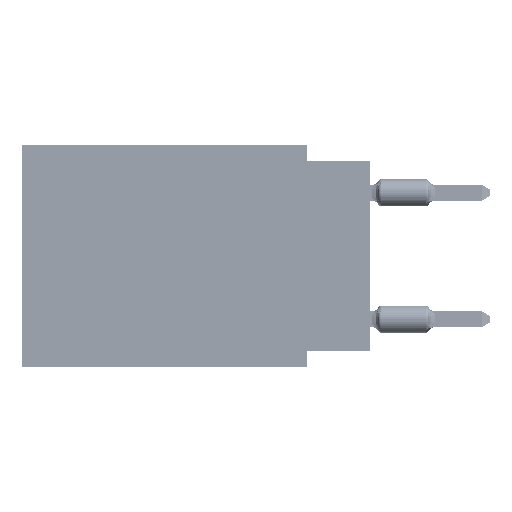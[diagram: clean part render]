
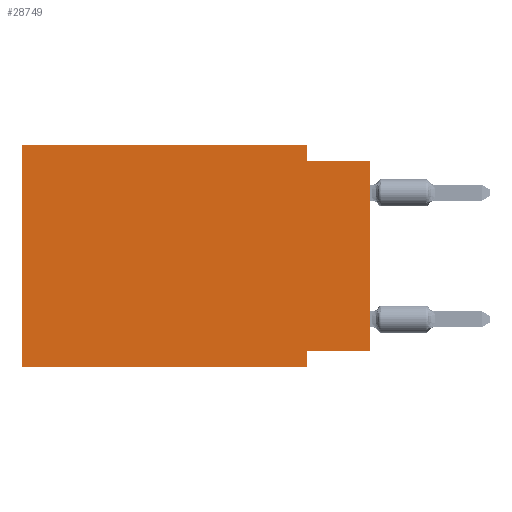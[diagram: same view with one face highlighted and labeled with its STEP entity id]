
A CAD part, left-side view. The second image highlights one B-rep face of the part: STEP entity #28749.
In plain terms, the highlighted planar face has unit normal (-1, 0, 0).
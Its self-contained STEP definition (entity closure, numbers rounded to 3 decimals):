
#2673 = CARTESIAN_POINT ( 'NONE',  ( 0., 13.97, 0. ) ) ;
#3300 = CARTESIAN_POINT ( 'NONE',  ( 0., 2.54, -8.89 ) ) ;
#5452 = LINE ( 'NONE', #49306, #40307 ) ;
#6065 = CARTESIAN_POINT ( 'NONE',  ( 0., 0., -8.255 ) ) ;
#8276 = EDGE_CURVE ( 'NONE', #54910, #14964, #117105, .T. ) ;
#8331 = VECTOR ( 'NONE', #71181, 1000. ) ;
#9939 = EDGE_CURVE ( 'NONE', #44845, #18019, #48872, .T. ) ;
#13936 = DIRECTION ( 'NONE',  ( 0., 0., -1. ) ) ;
#14964 = VERTEX_POINT ( 'NONE', #2673 ) ;
#15237 = CARTESIAN_POINT ( 'NONE',  ( 0., 2.54, -8.89 ) ) ;
#16315 = VERTEX_POINT ( 'NONE', #67379 ) ;
#18019 = VERTEX_POINT ( 'NONE', #29750 ) ;
#19288 = CARTESIAN_POINT ( 'NONE',  ( 0., 0., -0.635 ) ) ;
#24327 = PLANE ( 'NONE',  #94145 ) ;
#25534 = CARTESIAN_POINT ( 'NONE',  ( 0., 0., 0. ) ) ;
#26233 = VERTEX_POINT ( 'NONE', #15237 ) ;
#27404 = DIRECTION ( 'NONE',  ( 0., 1., 0. ) ) ;
#28749 = ADVANCED_FACE ( 'NONE', ( #51570 ), #24327, .F. ) ;
#29750 = CARTESIAN_POINT ( 'NONE',  ( 0., 0., -0.635 ) ) ;
#32771 = CARTESIAN_POINT ( 'NONE',  ( 0., 13.97, -8.89 ) ) ;
#34827 = ORIENTED_EDGE ( 'NONE', *, *, #89122, .F. ) ;
#35045 = CARTESIAN_POINT ( 'NONE',  ( 0., 13.97, 0. ) ) ;
#36717 = DIRECTION ( 'NONE',  ( 0., 0., 1. ) ) ;
#38510 = ORIENTED_EDGE ( 'NONE', *, *, #9939, .F. ) ;
#38607 = LINE ( 'NONE', #47521, #50872 ) ;
#40307 = VECTOR ( 'NONE', #59360, 1000. ) ;
#40900 = CARTESIAN_POINT ( 'NONE',  ( 0., 13.97, 0. ) ) ;
#44845 = VERTEX_POINT ( 'NONE', #47089 ) ;
#47089 = CARTESIAN_POINT ( 'NONE',  ( 0., 2.54, -0.635 ) ) ;
#47521 = CARTESIAN_POINT ( 'NONE',  ( 0., 0., -8.255 ) ) ;
#47622 = EDGE_CURVE ( 'NONE', #99064, #44845, #5452, .T. ) ;
#48186 = ORIENTED_EDGE ( 'NONE', *, *, #61670, .T. ) ;
#48872 = LINE ( 'NONE', #19288, #99717 ) ;
#49306 = CARTESIAN_POINT ( 'NONE',  ( 0., 2.54, 0. ) ) ;
#50872 = VECTOR ( 'NONE', #27404, 1000. ) ;
#51570 = FACE_OUTER_BOUND ( 'NONE', #85907, .T. ) ;
#52399 = VECTOR ( 'NONE', #115671, 1000. ) ;
#53425 = LINE ( 'NONE', #35045, #8331 ) ;
#54518 = LINE ( 'NONE', #25534, #69589 ) ;
#54910 = VERTEX_POINT ( 'NONE', #92592 ) ;
#59360 = DIRECTION ( 'NONE',  ( 0., 0., -1. ) ) ;
#61670 = EDGE_CURVE ( 'NONE', #88846, #18019, #54518, .T. ) ;
#63228 = CARTESIAN_POINT ( 'NONE',  ( 0., 13.97, 0. ) ) ;
#66443 = ORIENTED_EDGE ( 'NONE', *, *, #90180, .F. ) ;
#67121 = VECTOR ( 'NONE', #98190, 1000. ) ;
#67379 = CARTESIAN_POINT ( 'NONE',  ( 0., 2.54, -8.255 ) ) ;
#69329 = DIRECTION ( 'NONE',  ( 0., 0., -1. ) ) ;
#69589 = VECTOR ( 'NONE', #36717, 1000. ) ;
#70048 = ORIENTED_EDGE ( 'NONE', *, *, #96653, .F. ) ;
#71181 = DIRECTION ( 'NONE',  ( 0., -1., 0. ) ) ;
#74978 = LINE ( 'NONE', #3300, #89832 ) ;
#85907 = EDGE_LOOP ( 'NONE', ( #48186, #38510, #97736, #34827, #115506, #116827, #66443, #70048 ) ) ;
#88054 = CARTESIAN_POINT ( 'NONE',  ( 0., 2.54, 0. ) ) ;
#88846 = VERTEX_POINT ( 'NONE', #6065 ) ;
#89122 = EDGE_CURVE ( 'NONE', #14964, #99064, #53425, .T. ) ;
#89832 = VECTOR ( 'NONE', #13936, 1000. ) ;
#90180 = EDGE_CURVE ( 'NONE', #16315, #26233, #74978, .T. ) ;
#92592 = CARTESIAN_POINT ( 'NONE',  ( 0., 13.97, -8.89 ) ) ;
#94145 = AXIS2_PLACEMENT_3D ( 'NONE', #40900, #104291, #69329 ) ;
#96653 = EDGE_CURVE ( 'NONE', #88846, #16315, #38607, .T. ) ;
#97736 = ORIENTED_EDGE ( 'NONE', *, *, #47622, .F. ) ;
#98190 = DIRECTION ( 'NONE',  ( 0., 0., 1. ) ) ;
#99064 = VERTEX_POINT ( 'NONE', #88054 ) ;
#99717 = VECTOR ( 'NONE', #100999, 1000. ) ;
#100999 = DIRECTION ( 'NONE',  ( 0., -1., 0. ) ) ;
#104291 = DIRECTION ( 'NONE',  ( 1., 0., 0. ) ) ;
#105708 = EDGE_CURVE ( 'NONE', #54910, #26233, #113911, .T. ) ;
#113911 = LINE ( 'NONE', #32771, #52399 ) ;
#115506 = ORIENTED_EDGE ( 'NONE', *, *, #8276, .F. ) ;
#115671 = DIRECTION ( 'NONE',  ( 0., -1., 0. ) ) ;
#116827 = ORIENTED_EDGE ( 'NONE', *, *, #105708, .T. ) ;
#117105 = LINE ( 'NONE', #63228, #67121 ) ;
